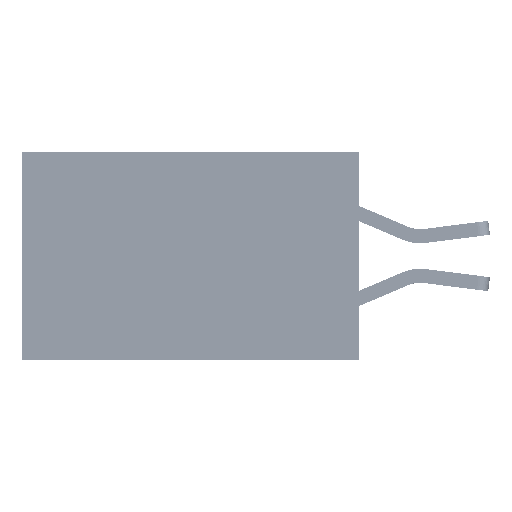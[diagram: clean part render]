
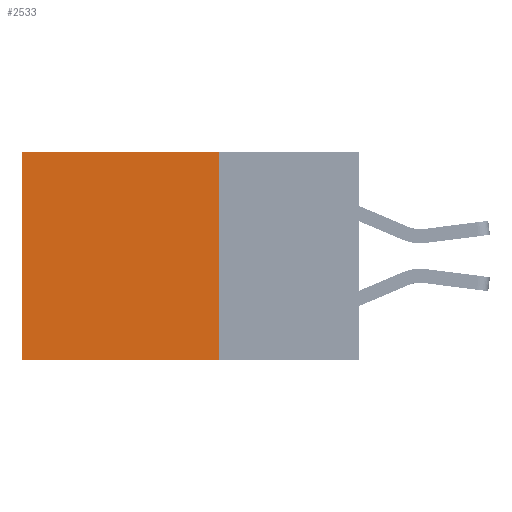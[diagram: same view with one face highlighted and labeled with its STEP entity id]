
A CAD part, left-side view. The second image highlights one B-rep face of the part: STEP entity #2533.
In plain terms, the highlighted planar face has unit normal (-1, 0, 0).
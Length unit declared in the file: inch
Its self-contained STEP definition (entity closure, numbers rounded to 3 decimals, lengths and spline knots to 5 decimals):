
#208 = CARTESIAN_POINT ( 'NONE',  ( 0.2875, 0.6, 0. ) ) ;
#950 = CARTESIAN_POINT ( 'NONE',  ( 0.2875, 0.6, -0.37 ) ) ;
#1047 = ORIENTED_EDGE ( 'NONE', *, *, #24609, .T. ) ;
#1940 = LINE ( 'NONE', #208, #5566 ) ;
#2533 = ADVANCED_FACE ( 'NONE', ( #32307 ), #28903, .F. ) ;
#2697 = LINE ( 'NONE', #32177, #9694 ) ;
#4698 = VERTEX_POINT ( 'NONE', #40416 ) ;
#5566 = VECTOR ( 'NONE', #13038, 39.37008 ) ;
#6666 = DIRECTION ( 'NONE',  ( 0., 0., -1. ) ) ;
#8325 = EDGE_CURVE ( 'NONE', #4698, #40660, #8404, .T. ) ;
#8404 = LINE ( 'NONE', #14819, #33449 ) ;
#8820 = ORIENTED_EDGE ( 'NONE', *, *, #21672, .T. ) ;
#9694 = VECTOR ( 'NONE', #18744, 39.37008 ) ;
#9874 = CARTESIAN_POINT ( 'NONE',  ( 0.2875, 0.25, 0. ) ) ;
#10625 = DIRECTION ( 'NONE',  ( 0., 0., -1. ) ) ;
#13038 = DIRECTION ( 'NONE',  ( 0., 0., -1. ) ) ;
#14819 = CARTESIAN_POINT ( 'NONE',  ( 0.2875, 0.25, -0.37 ) ) ;
#14845 = CARTESIAN_POINT ( 'NONE',  ( 0.2875, 0.6, 0. ) ) ;
#18744 = DIRECTION ( 'NONE',  ( 0., 1., 0. ) ) ;
#19276 = ORIENTED_EDGE ( 'NONE', *, *, #24197, .F. ) ;
#20460 = CARTESIAN_POINT ( 'NONE',  ( 0.2875, 0.25, 0. ) ) ;
#21442 = DIRECTION ( 'NONE',  ( 0., 1., 0. ) ) ;
#21672 = EDGE_CURVE ( 'NONE', #39008, #40660, #1940, .T. ) ;
#23859 = EDGE_LOOP ( 'NONE', ( #8820, #36745, #19276, #1047 ) ) ;
#24197 = EDGE_CURVE ( 'NONE', #34804, #4698, #33267, .T. ) ;
#24609 = EDGE_CURVE ( 'NONE', #34804, #39008, #2697, .T. ) ;
#25240 = CARTESIAN_POINT ( 'NONE',  ( 0.2875, 0.25, 0. ) ) ;
#28903 = PLANE ( 'NONE',  #33343 ) ;
#32172 = VECTOR ( 'NONE', #10625, 39.37008 ) ;
#32177 = CARTESIAN_POINT ( 'NONE',  ( 0.2875, 0.25, 0. ) ) ;
#32307 = FACE_OUTER_BOUND ( 'NONE', #23859, .T. ) ;
#33267 = LINE ( 'NONE', #20460, #32172 ) ;
#33343 = AXIS2_PLACEMENT_3D ( 'NONE', #9874, #35920, #6666 ) ;
#33449 = VECTOR ( 'NONE', #21442, 39.37008 ) ;
#34804 = VERTEX_POINT ( 'NONE', #25240 ) ;
#35920 = DIRECTION ( 'NONE',  ( 1., 0., 0. ) ) ;
#36745 = ORIENTED_EDGE ( 'NONE', *, *, #8325, .F. ) ;
#39008 = VERTEX_POINT ( 'NONE', #14845 ) ;
#40416 = CARTESIAN_POINT ( 'NONE',  ( 0.2875, 0.25, -0.37 ) ) ;
#40660 = VERTEX_POINT ( 'NONE', #950 ) ;
